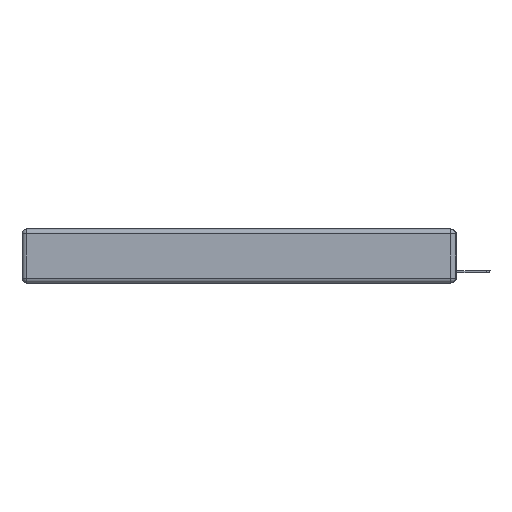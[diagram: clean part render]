
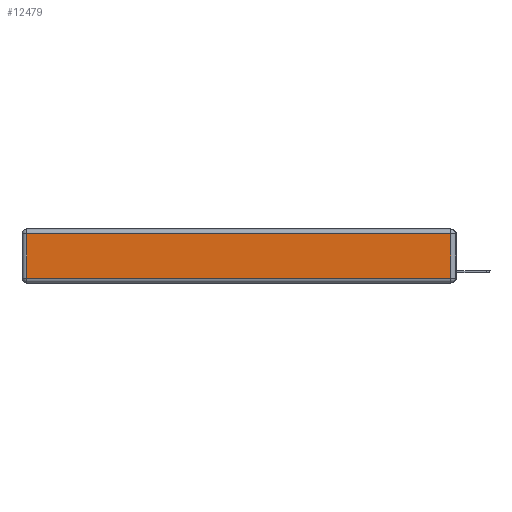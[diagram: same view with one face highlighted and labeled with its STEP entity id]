
A CAD part, left-side view. The second image highlights one B-rep face of the part: STEP entity #12479.
In plain terms, the highlighted planar face has unit normal (-1, 0, 0).
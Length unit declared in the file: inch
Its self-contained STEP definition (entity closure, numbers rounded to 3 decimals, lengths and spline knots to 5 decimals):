
#954 = LINE ( 'NONE', #11131, #18825 ) ;
#1314 = AXIS2_PLACEMENT_3D ( 'NONE', #19941, #3918, #5633 ) ;
#2037 = VERTEX_POINT ( 'NONE', #10385 ) ;
#2073 = VECTOR ( 'NONE', #12041, 39.37008 ) ;
#2304 = EDGE_LOOP ( 'NONE', ( #21612, #5060, #18376, #21196 ) ) ;
#2669 = PLANE ( 'NONE',  #1314 ) ;
#2781 = LINE ( 'NONE', #11713, #20037 ) ;
#2826 = EDGE_CURVE ( 'NONE', #2037, #21830, #2781, .T. ) ;
#3918 = DIRECTION ( 'NONE',  ( -1., 0., 0. ) ) ;
#4932 = LINE ( 'NONE', #10435, #2073 ) ;
#5060 = ORIENTED_EDGE ( 'NONE', *, *, #5063, .T. ) ;
#5063 = EDGE_CURVE ( 'NONE', #21830, #21009, #21718, .T. ) ;
#5633 = DIRECTION ( 'NONE',  ( 0., 0., 1. ) ) ;
#10385 = CARTESIAN_POINT ( 'NONE',  ( 0., 2.72, -0.313 ) ) ;
#10435 = CARTESIAN_POINT ( 'NONE',  ( 0., 2.75, -0.03 ) ) ;
#11131 = CARTESIAN_POINT ( 'NONE',  ( 0., 2.72, -0.343 ) ) ;
#11243 = DIRECTION ( 'NONE',  ( 0., 0., -1. ) ) ;
#11713 = CARTESIAN_POINT ( 'NONE',  ( 0., 0., -0.313 ) ) ;
#12041 = DIRECTION ( 'NONE',  ( 0., 1., 0. ) ) ;
#12446 = EDGE_CURVE ( 'NONE', #21913, #2037, #954, .T. ) ;
#12479 = ADVANCED_FACE ( 'NONE', ( #21318 ), #2669, .T. ) ;
#12915 = CARTESIAN_POINT ( 'NONE',  ( 0., 0.03, -0.343 ) ) ;
#13039 = CARTESIAN_POINT ( 'NONE',  ( 0., 0.03, -0.03 ) ) ;
#14118 = CARTESIAN_POINT ( 'NONE',  ( 0., 2.72, -0.03 ) ) ;
#14144 = EDGE_CURVE ( 'NONE', #21009, #21913, #4932, .T. ) ;
#16471 = DIRECTION ( 'NONE',  ( 0., 0., 1. ) ) ;
#17237 = CARTESIAN_POINT ( 'NONE',  ( 0., 0.03, -0.313 ) ) ;
#18341 = DIRECTION ( 'NONE',  ( 0., -1., 0. ) ) ;
#18376 = ORIENTED_EDGE ( 'NONE', *, *, #14144, .T. ) ;
#18825 = VECTOR ( 'NONE', #11243, 39.37008 ) ;
#19941 = CARTESIAN_POINT ( 'NONE',  ( 0., 0., -0.343 ) ) ;
#20037 = VECTOR ( 'NONE', #18341, 39.37008 ) ;
#21009 = VERTEX_POINT ( 'NONE', #13039 ) ;
#21159 = VECTOR ( 'NONE', #16471, 39.37008 ) ;
#21196 = ORIENTED_EDGE ( 'NONE', *, *, #12446, .T. ) ;
#21318 = FACE_OUTER_BOUND ( 'NONE', #2304, .T. ) ;
#21612 = ORIENTED_EDGE ( 'NONE', *, *, #2826, .T. ) ;
#21718 = LINE ( 'NONE', #12915, #21159 ) ;
#21830 = VERTEX_POINT ( 'NONE', #17237 ) ;
#21913 = VERTEX_POINT ( 'NONE', #14118 ) ;
